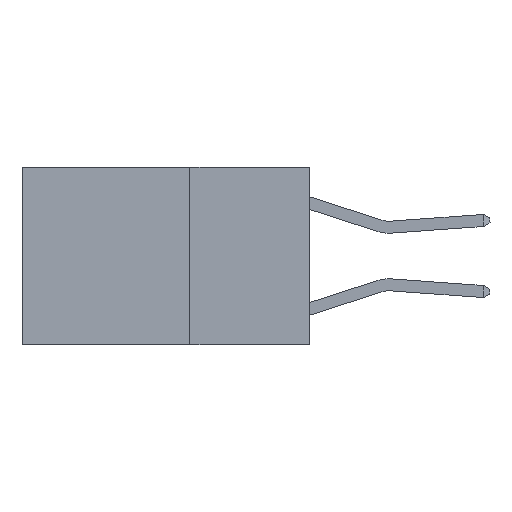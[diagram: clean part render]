
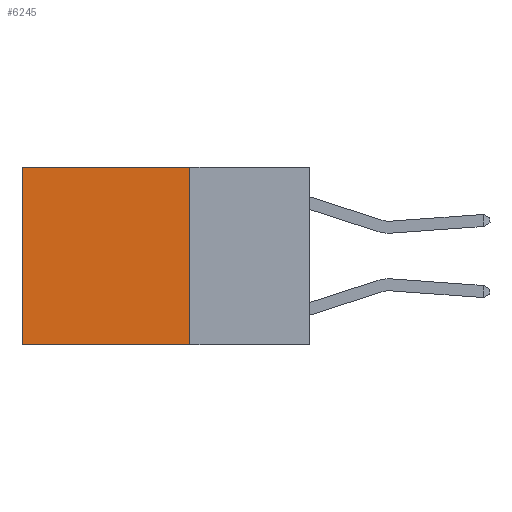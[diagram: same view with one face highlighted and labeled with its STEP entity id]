
A CAD part, left-side view. The second image highlights one B-rep face of the part: STEP entity #6245.
In plain terms, the highlighted planar face has unit normal (-1, 0, 0).
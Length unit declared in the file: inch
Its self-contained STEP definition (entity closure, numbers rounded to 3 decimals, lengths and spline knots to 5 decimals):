
#289 = ORIENTED_EDGE ( 'NONE', *, *, #12040, .F. ) ;
#529 = EDGE_CURVE ( 'NONE', #4946, #994, #3236, .T. ) ;
#893 = PLANE ( 'NONE',  #9607 ) ;
#994 = VERTEX_POINT ( 'NONE', #5140 ) ;
#1040 = CARTESIAN_POINT ( 'NONE',  ( 0.2625, 0.25, -0.37 ) ) ;
#1364 = CARTESIAN_POINT ( 'NONE',  ( 0.2625, 0.6, 0. ) ) ;
#1826 = VECTOR ( 'NONE', #8093, 39.37008 ) ;
#1861 = CARTESIAN_POINT ( 'NONE',  ( 0.2625, 0.25, 0. ) ) ;
#2095 = LINE ( 'NONE', #1364, #11177 ) ;
#2202 = ORIENTED_EDGE ( 'NONE', *, *, #529, .T. ) ;
#2505 = DIRECTION ( 'NONE',  ( 0., 0., -1. ) ) ;
#2710 = CARTESIAN_POINT ( 'NONE',  ( 0.2625, 0.25, 0. ) ) ;
#3085 = CARTESIAN_POINT ( 'NONE',  ( 0.2625, 0.25, 0. ) ) ;
#3236 = LINE ( 'NONE', #3085, #10029 ) ;
#3515 = LINE ( 'NONE', #2710, #7477 ) ;
#4946 = VERTEX_POINT ( 'NONE', #1861 ) ;
#5140 = CARTESIAN_POINT ( 'NONE',  ( 0.2625, 0.6, 0. ) ) ;
#5408 = CARTESIAN_POINT ( 'NONE',  ( 0.2625, 0.6, -0.37 ) ) ;
#5647 = CARTESIAN_POINT ( 'NONE',  ( 0.2625, 0.25, -0.37 ) ) ;
#5700 = ORIENTED_EDGE ( 'NONE', *, *, #7937, .F. ) ;
#6245 = ADVANCED_FACE ( 'NONE', ( #12182 ), #893, .F. ) ;
#6772 = DIRECTION ( 'NONE',  ( 0., 1., 0. ) ) ;
#7174 = DIRECTION ( 'NONE',  ( 0., 0., -1. ) ) ;
#7477 = VECTOR ( 'NONE', #2505, 39.37008 ) ;
#7808 = DIRECTION ( 'NONE',  ( 1., 0., 0. ) ) ;
#7937 = EDGE_CURVE ( 'NONE', #7987, #14205, #12346, .T. ) ;
#7987 = VERTEX_POINT ( 'NONE', #5647 ) ;
#8093 = DIRECTION ( 'NONE',  ( 0., 1., 0. ) ) ;
#9536 = EDGE_LOOP ( 'NONE', ( #13556, #5700, #289, #2202 ) ) ;
#9607 = AXIS2_PLACEMENT_3D ( 'NONE', #14374, #7808, #11039 ) ;
#10029 = VECTOR ( 'NONE', #6772, 39.37008 ) ;
#11039 = DIRECTION ( 'NONE',  ( 0., 0., -1. ) ) ;
#11177 = VECTOR ( 'NONE', #7174, 39.37008 ) ;
#11316 = EDGE_CURVE ( 'NONE', #994, #14205, #2095, .T. ) ;
#12040 = EDGE_CURVE ( 'NONE', #4946, #7987, #3515, .T. ) ;
#12182 = FACE_OUTER_BOUND ( 'NONE', #9536, .T. ) ;
#12346 = LINE ( 'NONE', #1040, #1826 ) ;
#13556 = ORIENTED_EDGE ( 'NONE', *, *, #11316, .T. ) ;
#14205 = VERTEX_POINT ( 'NONE', #5408 ) ;
#14374 = CARTESIAN_POINT ( 'NONE',  ( 0.2625, 0.25, 0. ) ) ;
